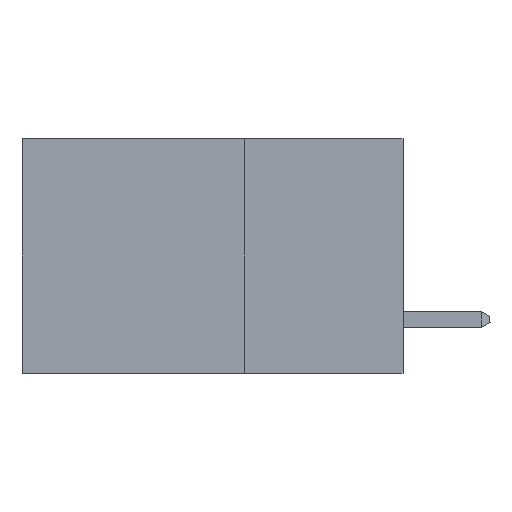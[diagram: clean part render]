
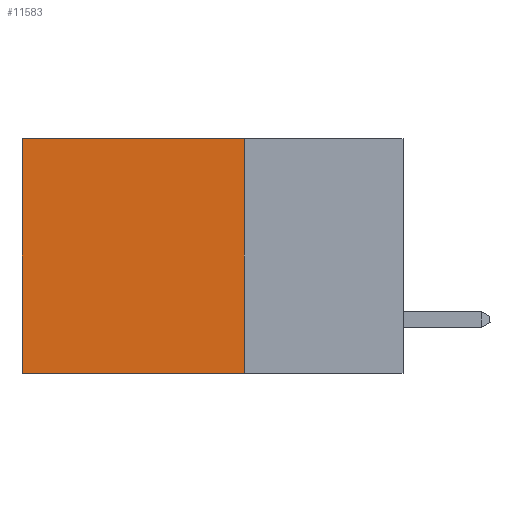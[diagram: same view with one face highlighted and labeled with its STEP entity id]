
A CAD part, left-side view. The second image highlights one B-rep face of the part: STEP entity #11583.
In plain terms, the highlighted planar face has unit normal (-1, 0, 0).
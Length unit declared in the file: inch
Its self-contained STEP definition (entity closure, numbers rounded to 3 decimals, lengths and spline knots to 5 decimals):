
#1089 = ORIENTED_EDGE ( 'NONE', *, *, #4759, .F. ) ;
#2071 = DIRECTION ( 'NONE',  ( 0., 1., 0. ) ) ;
#3190 = DIRECTION ( 'NONE',  ( 0., 1., 0. ) ) ;
#4520 = FACE_OUTER_BOUND ( 'NONE', #22096, .T. ) ;
#4759 = EDGE_CURVE ( 'NONE', #5207, #15498, #14340, .T. ) ;
#5207 = VERTEX_POINT ( 'NONE', #13470 ) ;
#5864 = ORIENTED_EDGE ( 'NONE', *, *, #17542, .F. ) ;
#6225 = CARTESIAN_POINT ( 'NONE',  ( 0.2875, 0.25, 0. ) ) ;
#6763 = VECTOR ( 'NONE', #21054, 39.37008 ) ;
#7244 = VERTEX_POINT ( 'NONE', #13955 ) ;
#7258 = VECTOR ( 'NONE', #17990, 39.37008 ) ;
#7808 = LINE ( 'NONE', #21567, #7258 ) ;
#7994 = PLANE ( 'NONE',  #12696 ) ;
#8239 = ORIENTED_EDGE ( 'NONE', *, *, #23537, .T. ) ;
#8257 = EDGE_CURVE ( 'NONE', #7244, #15498, #7808, .T. ) ;
#8904 = LINE ( 'NONE', #12141, #22846 ) ;
#10196 = LINE ( 'NONE', #18975, #6763 ) ;
#10596 = ORIENTED_EDGE ( 'NONE', *, *, #8257, .T. ) ;
#11583 = ADVANCED_FACE ( 'NONE', ( #4520 ), #7994, .F. ) ;
#12141 = CARTESIAN_POINT ( 'NONE',  ( 0.2875, 0.25, 0. ) ) ;
#12338 = CARTESIAN_POINT ( 'NONE',  ( 0.2875, 0.25, -0.37 ) ) ;
#12696 = AXIS2_PLACEMENT_3D ( 'NONE', #6225, #15362, #18905 ) ;
#13470 = CARTESIAN_POINT ( 'NONE',  ( 0.2875, 0.25, -0.37 ) ) ;
#13955 = CARTESIAN_POINT ( 'NONE',  ( 0.2875, 0.6, 0. ) ) ;
#14340 = LINE ( 'NONE', #12338, #15175 ) ;
#15175 = VECTOR ( 'NONE', #2071, 39.37008 ) ;
#15362 = DIRECTION ( 'NONE',  ( 1., 0., 0. ) ) ;
#15498 = VERTEX_POINT ( 'NONE', #20567 ) ;
#17542 = EDGE_CURVE ( 'NONE', #21469, #5207, #10196, .T. ) ;
#17990 = DIRECTION ( 'NONE',  ( 0., 0., -1. ) ) ;
#18905 = DIRECTION ( 'NONE',  ( 0., 0., -1. ) ) ;
#18975 = CARTESIAN_POINT ( 'NONE',  ( 0.2875, 0.25, 0. ) ) ;
#20352 = CARTESIAN_POINT ( 'NONE',  ( 0.2875, 0.25, 0. ) ) ;
#20567 = CARTESIAN_POINT ( 'NONE',  ( 0.2875, 0.6, -0.37 ) ) ;
#21054 = DIRECTION ( 'NONE',  ( 0., 0., -1. ) ) ;
#21469 = VERTEX_POINT ( 'NONE', #20352 ) ;
#21567 = CARTESIAN_POINT ( 'NONE',  ( 0.2875, 0.6, 0. ) ) ;
#22096 = EDGE_LOOP ( 'NONE', ( #10596, #1089, #5864, #8239 ) ) ;
#22846 = VECTOR ( 'NONE', #3190, 39.37008 ) ;
#23537 = EDGE_CURVE ( 'NONE', #21469, #7244, #8904, .T. ) ;
